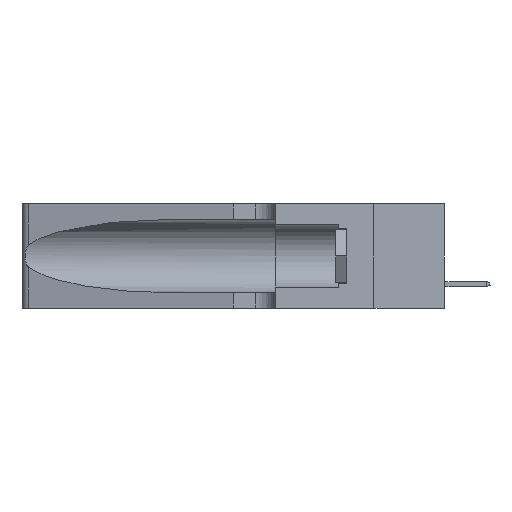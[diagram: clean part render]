
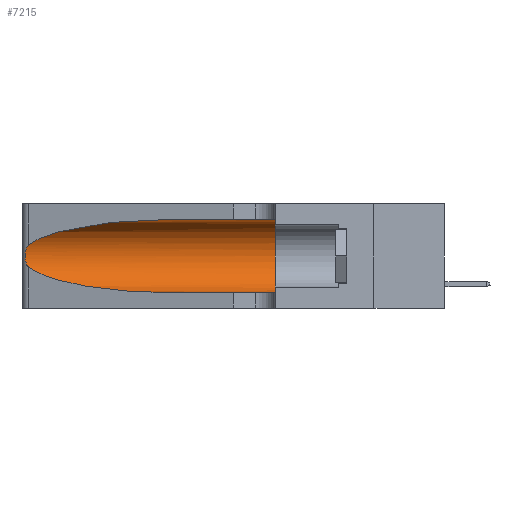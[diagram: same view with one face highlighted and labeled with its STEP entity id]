
A CAD part, left-side view. The second image highlights one B-rep face of the part: STEP entity #7215.
In plain terms, the highlighted cylindrical face has radius 3.308 mm (diameter 6.617 mm), a partial arc.
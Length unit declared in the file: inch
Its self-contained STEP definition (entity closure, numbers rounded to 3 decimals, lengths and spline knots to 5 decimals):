
#328 = CARTESIAN_POINT ( 'NONE',  ( 0.1305, 0.35, 0.185 ) ) ;
#486 =( BOUNDED_CURVE ( )  B_SPLINE_CURVE ( 3, ( #7637, #10927, #17541, #36985 ),
 .UNSPECIFIED., .F., .F. ) 
 B_SPLINE_CURVE_WITH_KNOTS ( ( 4, 4 ),
 ( 1.5708, 2.84003 ),
 .UNSPECIFIED. ) 
 CURVE ( )  GEOMETRIC_REPRESENTATION_ITEM ( )  RATIONAL_B_SPLINE_CURVE ( ( 1., 0.87, 0.87, 1. ) ) 
 REPRESENTATION_ITEM ( '' )  );
#2868 = CARTESIAN_POINT ( 'NONE',  ( 0.26018, 1.23835, 0.19895 ) ) ;
#3008 = CARTESIAN_POINT ( 'NONE',  ( 0.25639, 1.23186, 0.15144 ) ) ;
#3699 = DIRECTION ( 'NONE',  ( 0., 0., -1. ) ) ;
#5570 = ORIENTED_EDGE ( 'NONE', *, *, #22729, .F. ) ;
#7215 = ADVANCED_FACE ( 'NONE', ( #8773 ), #11360, .F. ) ;
#7611 = CARTESIAN_POINT ( 'NONE',  ( 0.25487, 1.22718, 0.14631 ) ) ;
#7637 = CARTESIAN_POINT ( 'NONE',  ( 0.1305, 0.72297, 0.31525 ) ) ;
#8773 = FACE_OUTER_BOUND ( 'NONE', #38869, .T. ) ;
#9439 = CARTESIAN_POINT ( 'NONE',  ( 0.26075, 1.23896, 0.19203 ) ) ;
#10431 = CARTESIAN_POINT ( 'NONE',  ( 0.1305, 0.35, 0.05475 ) ) ;
#10445 =( BOUNDED_CURVE ( )  B_SPLINE_CURVE ( 3, ( #39353, #20366, #36265, #35980 ),
 .UNSPECIFIED., .F., .F. ) 
 B_SPLINE_CURVE_WITH_KNOTS ( ( 4, 4 ),
 ( 3.44316, 4.71239 ),
 .UNSPECIFIED. ) 
 CURVE ( )  GEOMETRIC_REPRESENTATION_ITEM ( )  RATIONAL_B_SPLINE_CURVE ( ( 1., 0.87, 0.87, 1. ) ) 
 REPRESENTATION_ITEM ( '' )  );
#10927 = CARTESIAN_POINT ( 'NONE',  ( 0.18966, 0.96281, 0.31525 ) ) ;
#11057 = AXIS2_PLACEMENT_3D ( 'NONE', #15023, #25679, #3699 ) ;
#11360 = CYLINDRICAL_SURFACE ( 'NONE', #11057, 0.13025 ) ;
#12338 = EDGE_CURVE ( 'NONE', #26430, #18817, #39892, .T. ) ;
#12742 = ORIENTED_EDGE ( 'NONE', *, *, #12338, .T. ) ;
#15023 = CARTESIAN_POINT ( 'NONE',  ( 0.1305, 1.61858, 0.185 ) ) ;
#15467 = EDGE_CURVE ( 'NONE', #16605, #22511, #20437, .T. ) ;
#15634 = CARTESIAN_POINT ( 'NONE',  ( 0.25555, 1.22994, 0.2215 ) ) ;
#15696 = LINE ( 'NONE', #30234, #20263 ) ;
#15917 = CARTESIAN_POINT ( 'NONE',  ( 0.25856, 1.23593, 0.16098 ) ) ;
#15945 = ORIENTED_EDGE ( 'NONE', *, *, #15467, .T. ) ;
#16055 = CARTESIAN_POINT ( 'NONE',  ( 0.1305, 1.61858, 0.05475 ) ) ;
#16605 = VERTEX_POINT ( 'NONE', #29034 ) ;
#17541 = CARTESIAN_POINT ( 'NONE',  ( 0.2373, 1.15595, 0.28018 ) ) ;
#17962 = ORIENTED_EDGE ( 'NONE', *, *, #28723, .F. ) ;
#18817 = VERTEX_POINT ( 'NONE', #7611 ) ;
#19163 = CARTESIAN_POINT ( 'NONE',  ( 0.25487, 1.22718, 0.22369 ) ) ;
#20010 = CARTESIAN_POINT ( 'NONE',  ( 0.25555, 1.22993, 0.14849 ) ) ;
#20263 = VECTOR ( 'NONE', #30780, 39.37008 ) ;
#20366 = CARTESIAN_POINT ( 'NONE',  ( 0.2373, 1.15595, 0.08982 ) ) ;
#20437 = LINE ( 'NONE', #16055, #30510 ) ;
#20691 = VERTEX_POINT ( 'NONE', #38720 ) ;
#22422 = CARTESIAN_POINT ( 'NONE',  ( 0.25789, 1.23486, 0.15765 ) ) ;
#22511 = VERTEX_POINT ( 'NONE', #10431 ) ;
#22729 = EDGE_CURVE ( 'NONE', #20691, #22511, #26124, .T. ) ;
#23423 = CARTESIAN_POINT ( 'NONE',  ( 0.1305, 0.72297, 0.31525 ) ) ;
#25679 = DIRECTION ( 'NONE',  ( 0., -1., 0. ) ) ;
#26124 = CIRCLE ( 'NONE', #40564, 0.13025 ) ;
#26430 = VERTEX_POINT ( 'NONE', #32190 ) ;
#28481 = CARTESIAN_POINT ( 'NONE',  ( 0.25639, 1.23184, 0.21858 ) ) ;
#28685 = ORIENTED_EDGE ( 'NONE', *, *, #28699, .T. ) ;
#28699 = EDGE_CURVE ( 'NONE', #32059, #26430, #486, .T. ) ;
#28723 = EDGE_CURVE ( 'NONE', #32059, #20691, #15696, .T. ) ;
#28759 = CARTESIAN_POINT ( 'NONE',  ( 0.25854, 1.2359, 0.20912 ) ) ;
#29033 = DIRECTION ( 'NONE',  ( 0., -1., 0. ) ) ;
#29034 = CARTESIAN_POINT ( 'NONE',  ( 0.1305, 0.72297, 0.05475 ) ) ;
#29505 = DIRECTION ( 'NONE',  ( 0., 0., 1. ) ) ;
#30234 = CARTESIAN_POINT ( 'NONE',  ( 0.1305, 1.61858, 0.31525 ) ) ;
#30510 = VECTOR ( 'NONE', #29033, 39.37008 ) ;
#30780 = DIRECTION ( 'NONE',  ( 0., -1., 0. ) ) ;
#31994 = CARTESIAN_POINT ( 'NONE',  ( 0.26075, 1.23896, 0.178 ) ) ;
#32059 = VERTEX_POINT ( 'NONE', #23423 ) ;
#32190 = CARTESIAN_POINT ( 'NONE',  ( 0.25487, 1.22718, 0.22369 ) ) ;
#32829 = CARTESIAN_POINT ( 'NONE',  ( 0.25487, 1.22718, 0.14631 ) ) ;
#34474 = EDGE_CURVE ( 'NONE', #18817, #16605, #10445, .T. ) ;
#35080 = CARTESIAN_POINT ( 'NONE',  ( 0.25787, 1.23484, 0.2124 ) ) ;
#35205 = CARTESIAN_POINT ( 'NONE',  ( 0.26017, 1.23833, 0.17102 ) ) ;
#35980 = CARTESIAN_POINT ( 'NONE',  ( 0.1305, 0.72297, 0.05475 ) ) ;
#36265 = CARTESIAN_POINT ( 'NONE',  ( 0.18966, 0.96281, 0.05475 ) ) ;
#36985 = CARTESIAN_POINT ( 'NONE',  ( 0.25487, 1.22718, 0.22369 ) ) ;
#38720 = CARTESIAN_POINT ( 'NONE',  ( 0.1305, 0.35, 0.31525 ) ) ;
#38869 = EDGE_LOOP ( 'NONE', ( #28685, #12742, #40910, #15945, #5570, #17962 ) ) ;
#39062 = DIRECTION ( 'NONE',  ( 0., 1., 0. ) ) ;
#39353 = CARTESIAN_POINT ( 'NONE',  ( 0.25487, 1.22718, 0.14631 ) ) ;
#39892 = B_SPLINE_CURVE_WITH_KNOTS ( 'NONE', 3,
 ( #19163, #15634, #28481, #35080, #28759, #2868, #9439, #31994, #35205, #15917, #22422, #3008, #20010, #32829 ),
 .UNSPECIFIED., .F., .F.,
 ( 4, 2, 2, 2, 2, 2, 4 ),
 ( 0., 0.00027, 0.00053, 0.00107, 0.0016, 0.00187, 0.00214 ),
 .UNSPECIFIED. ) ;
#40564 = AXIS2_PLACEMENT_3D ( 'NONE', #328, #39062, #29505 ) ;
#40910 = ORIENTED_EDGE ( 'NONE', *, *, #34474, .T. ) ;
